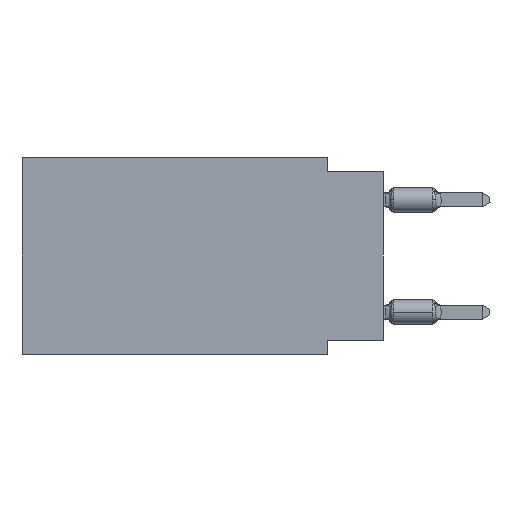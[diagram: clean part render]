
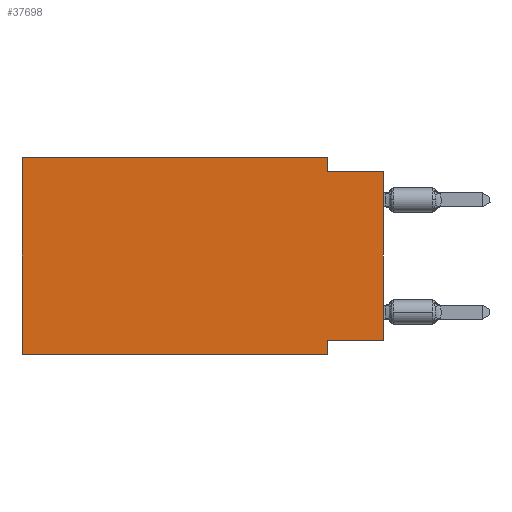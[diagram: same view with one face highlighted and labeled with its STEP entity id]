
A CAD part, left-side view. The second image highlights one B-rep face of the part: STEP entity #37698.
In plain terms, the highlighted planar face has unit normal (-1, 0, 0).
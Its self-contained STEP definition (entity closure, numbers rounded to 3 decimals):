
#51 = VECTOR ( 'NONE', #17219, 1000. ) ;
#725 = DIRECTION ( 'NONE',  ( 1., 0., 0. ) ) ;
#1080 = VECTOR ( 'NONE', #18646, 1000. ) ;
#1238 = LINE ( 'NONE', #10160, #32615 ) ;
#1708 = VERTEX_POINT ( 'NONE', #20739 ) ;
#2100 = ORIENTED_EDGE ( 'NONE', *, *, #17133, .F. ) ;
#3807 = DIRECTION ( 'NONE',  ( 0., -1., 0. ) ) ;
#4590 = VERTEX_POINT ( 'NONE', #11429 ) ;
#6552 = CARTESIAN_POINT ( 'NONE',  ( 0., 0., -8.255 ) ) ;
#7167 = VECTOR ( 'NONE', #31257, 1000. ) ;
#7639 = DIRECTION ( 'NONE',  ( 0., 0., -1. ) ) ;
#8180 = ORIENTED_EDGE ( 'NONE', *, *, #38401, .T. ) ;
#8620 = CARTESIAN_POINT ( 'NONE',  ( 0., 16.383, 0. ) ) ;
#9686 = EDGE_CURVE ( 'NONE', #10308, #35176, #16768, .T. ) ;
#10160 = CARTESIAN_POINT ( 'NONE',  ( 0., 0., -0.635 ) ) ;
#10308 = VERTEX_POINT ( 'NONE', #12588 ) ;
#10792 = CARTESIAN_POINT ( 'NONE',  ( 0., 2.54, -8.255 ) ) ;
#11169 = EDGE_LOOP ( 'NONE', ( #8180, #37121, #16790, #16478, #17077, #31501, #2100, #31016 ) ) ;
#11429 = CARTESIAN_POINT ( 'NONE',  ( 0., 2.54, -0.635 ) ) ;
#11690 = CARTESIAN_POINT ( 'NONE',  ( 0., 2.54, 0. ) ) ;
#11693 = CARTESIAN_POINT ( 'NONE',  ( 0., 0., 0. ) ) ;
#11846 = VECTOR ( 'NONE', #23100, 1000. ) ;
#12296 = VECTOR ( 'NONE', #7639, 1000. ) ;
#12442 = VERTEX_POINT ( 'NONE', #37738 ) ;
#12588 = CARTESIAN_POINT ( 'NONE',  ( 0., 16.383, -8.89 ) ) ;
#14831 = EDGE_CURVE ( 'NONE', #18232, #34602, #33721, .T. ) ;
#15091 = CARTESIAN_POINT ( 'NONE',  ( 0., 16.383, 0. ) ) ;
#15207 = DIRECTION ( 'NONE',  ( 0., 0., -1. ) ) ;
#16478 = ORIENTED_EDGE ( 'NONE', *, *, #19897, .F. ) ;
#16584 = EDGE_CURVE ( 'NONE', #10308, #29424, #30174, .T. ) ;
#16768 = LINE ( 'NONE', #19159, #7167 ) ;
#16790 = ORIENTED_EDGE ( 'NONE', *, *, #22866, .F. ) ;
#17077 = ORIENTED_EDGE ( 'NONE', *, *, #16584, .F. ) ;
#17112 = VECTOR ( 'NONE', #35873, 1000. ) ;
#17133 = EDGE_CURVE ( 'NONE', #34602, #35176, #37386, .T. ) ;
#17176 = CARTESIAN_POINT ( 'NONE',  ( 0., 0., -8.255 ) ) ;
#17219 = DIRECTION ( 'NONE',  ( 0., 0., -1. ) ) ;
#17426 = LINE ( 'NONE', #11690, #51 ) ;
#18232 = VERTEX_POINT ( 'NONE', #17176 ) ;
#18646 = DIRECTION ( 'NONE',  ( 0., 1., 0. ) ) ;
#19159 = CARTESIAN_POINT ( 'NONE',  ( 0., 16.383, -8.89 ) ) ;
#19897 = EDGE_CURVE ( 'NONE', #29424, #1708, #29835, .T. ) ;
#20642 = CARTESIAN_POINT ( 'NONE',  ( 0., 2.54, -8.89 ) ) ;
#20739 = CARTESIAN_POINT ( 'NONE',  ( 0., 2.54, 0. ) ) ;
#22456 = VECTOR ( 'NONE', #36888, 1000. ) ;
#22634 = FACE_OUTER_BOUND ( 'NONE', #11169, .T. ) ;
#22866 = EDGE_CURVE ( 'NONE', #1708, #4590, #17426, .T. ) ;
#23100 = DIRECTION ( 'NONE',  ( 0., -1., 0. ) ) ;
#28083 = EDGE_CURVE ( 'NONE', #4590, #12442, #1238, .T. ) ;
#28357 = AXIS2_PLACEMENT_3D ( 'NONE', #29526, #725, #15207 ) ;
#29424 = VERTEX_POINT ( 'NONE', #38119 ) ;
#29526 = CARTESIAN_POINT ( 'NONE',  ( 0., 16.383, 0. ) ) ;
#29835 = LINE ( 'NONE', #8620, #11846 ) ;
#30174 = LINE ( 'NONE', #15091, #22456 ) ;
#31016 = ORIENTED_EDGE ( 'NONE', *, *, #14831, .F. ) ;
#31257 = DIRECTION ( 'NONE',  ( 0., -1., 0. ) ) ;
#31501 = ORIENTED_EDGE ( 'NONE', *, *, #9686, .T. ) ;
#32615 = VECTOR ( 'NONE', #3807, 1000. ) ;
#33721 = LINE ( 'NONE', #6552, #1080 ) ;
#34602 = VERTEX_POINT ( 'NONE', #10792 ) ;
#34744 = PLANE ( 'NONE',  #28357 ) ;
#35176 = VERTEX_POINT ( 'NONE', #20642 ) ;
#35208 = CARTESIAN_POINT ( 'NONE',  ( 0., 2.54, -8.89 ) ) ;
#35873 = DIRECTION ( 'NONE',  ( 0., 0., 1. ) ) ;
#36888 = DIRECTION ( 'NONE',  ( 0., 0., 1. ) ) ;
#37121 = ORIENTED_EDGE ( 'NONE', *, *, #28083, .F. ) ;
#37386 = LINE ( 'NONE', #35208, #12296 ) ;
#37698 = ADVANCED_FACE ( 'NONE', ( #22634 ), #34744, .F. ) ;
#37738 = CARTESIAN_POINT ( 'NONE',  ( 0., 0., -0.635 ) ) ;
#38119 = CARTESIAN_POINT ( 'NONE',  ( 0., 16.383, 0. ) ) ;
#38401 = EDGE_CURVE ( 'NONE', #18232, #12442, #38851, .T. ) ;
#38851 = LINE ( 'NONE', #11693, #17112 ) ;
